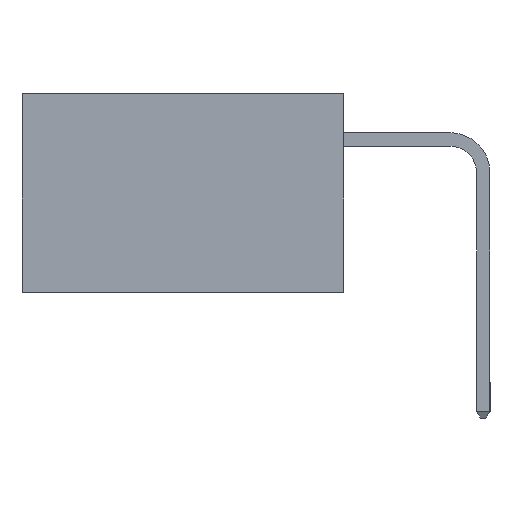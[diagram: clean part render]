
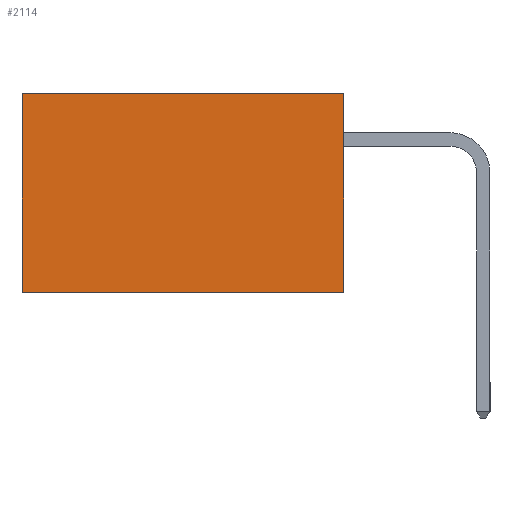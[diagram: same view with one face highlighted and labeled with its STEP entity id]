
A CAD part, left-side view. The second image highlights one B-rep face of the part: STEP entity #2114.
In plain terms, the highlighted planar face has unit normal (-1, 0, 0).
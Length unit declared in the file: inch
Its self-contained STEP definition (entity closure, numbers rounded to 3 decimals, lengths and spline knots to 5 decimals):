
#900 = DIRECTION ( 'NONE',  ( 0., 0., -1. ) ) ;
#1324 = DIRECTION ( 'NONE',  ( 0., 0., -1. ) ) ;
#1924 = ORIENTED_EDGE ( 'NONE', *, *, #13384, .T. ) ;
#2068 = CARTESIAN_POINT ( 'NONE',  ( 0.298, 0., -0.37 ) ) ;
#2114 = ADVANCED_FACE ( 'NONE', ( #11491 ), #8289, .F. ) ;
#2443 = VERTEX_POINT ( 'NONE', #3469 ) ;
#2682 = EDGE_CURVE ( 'NONE', #7278, #10115, #4483, .T. ) ;
#3243 = CARTESIAN_POINT ( 'NONE',  ( 0.298, 0., 0. ) ) ;
#3469 = CARTESIAN_POINT ( 'NONE',  ( 0.298, 0., -0.37 ) ) ;
#3477 = LINE ( 'NONE', #6291, #8575 ) ;
#3917 = VERTEX_POINT ( 'NONE', #4958 ) ;
#4142 = VECTOR ( 'NONE', #7899, 39.37008 ) ;
#4235 = VECTOR ( 'NONE', #900, 39.37008 ) ;
#4480 = CARTESIAN_POINT ( 'NONE',  ( 0.298, 0., 0. ) ) ;
#4483 = LINE ( 'NONE', #4480, #4142 ) ;
#4958 = CARTESIAN_POINT ( 'NONE',  ( 0.298, 0.6, -0.37 ) ) ;
#5205 = ORIENTED_EDGE ( 'NONE', *, *, #8468, .F. ) ;
#6291 = CARTESIAN_POINT ( 'NONE',  ( 0.298, 0., 0. ) ) ;
#6752 = LINE ( 'NONE', #7420, #4235 ) ;
#7053 = VECTOR ( 'NONE', #9673, 39.37008 ) ;
#7278 = VERTEX_POINT ( 'NONE', #3243 ) ;
#7420 = CARTESIAN_POINT ( 'NONE',  ( 0.298, 0.6, 0. ) ) ;
#7521 = EDGE_CURVE ( 'NONE', #7278, #2443, #3477, .T. ) ;
#7899 = DIRECTION ( 'NONE',  ( 0., 1., 0. ) ) ;
#8067 = ORIENTED_EDGE ( 'NONE', *, *, #7521, .F. ) ;
#8289 = PLANE ( 'NONE',  #12656 ) ;
#8468 = EDGE_CURVE ( 'NONE', #2443, #3917, #12367, .T. ) ;
#8537 = CARTESIAN_POINT ( 'NONE',  ( 0.298, 0.6, 0. ) ) ;
#8575 = VECTOR ( 'NONE', #12907, 39.37008 ) ;
#9293 = CARTESIAN_POINT ( 'NONE',  ( 0.298, 0., 0. ) ) ;
#9673 = DIRECTION ( 'NONE',  ( 0., 1., 0. ) ) ;
#10115 = VERTEX_POINT ( 'NONE', #8537 ) ;
#10887 = ORIENTED_EDGE ( 'NONE', *, *, #2682, .T. ) ;
#11491 = FACE_OUTER_BOUND ( 'NONE', #11834, .T. ) ;
#11656 = DIRECTION ( 'NONE',  ( 1., 0., 0. ) ) ;
#11834 = EDGE_LOOP ( 'NONE', ( #1924, #5205, #8067, #10887 ) ) ;
#12367 = LINE ( 'NONE', #2068, #7053 ) ;
#12656 = AXIS2_PLACEMENT_3D ( 'NONE', #9293, #11656, #1324 ) ;
#12907 = DIRECTION ( 'NONE',  ( 0., 0., -1. ) ) ;
#13384 = EDGE_CURVE ( 'NONE', #10115, #3917, #6752, .T. ) ;
